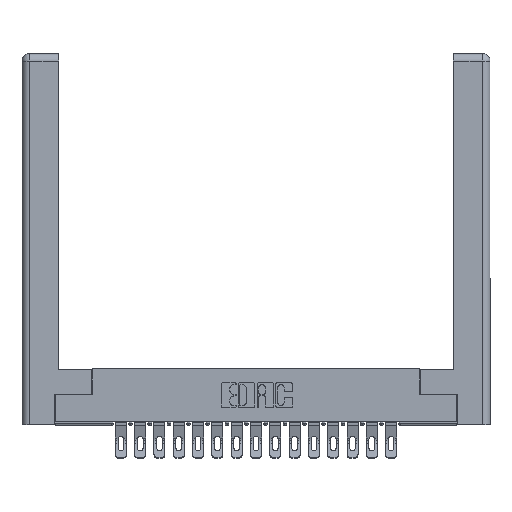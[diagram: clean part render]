
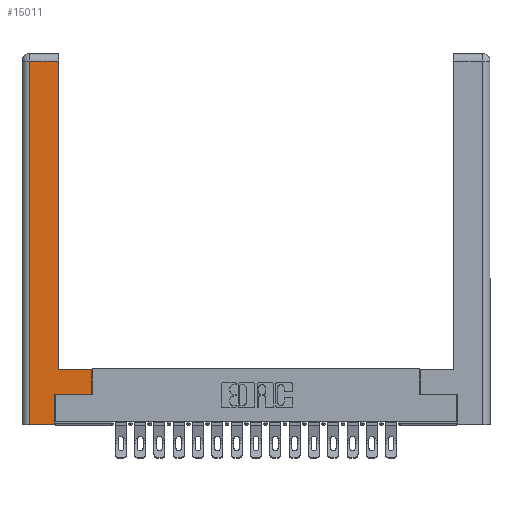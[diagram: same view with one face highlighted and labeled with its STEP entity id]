
A CAD part, top view. The second image highlights one B-rep face of the part: STEP entity #15011.
In plain terms, the highlighted planar face has unit normal (0, 0, 1).
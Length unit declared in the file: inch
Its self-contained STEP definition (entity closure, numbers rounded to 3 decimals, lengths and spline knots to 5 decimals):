
#7 = LINE ( 'NONE', #7671, #4098 ) ;
#144 = VECTOR ( 'NONE', #14500, 39.37008 ) ;
#373 = CARTESIAN_POINT ( 'NONE',  ( 0.565, 0.245, 0. ) ) ;
#655 = VERTEX_POINT ( 'NONE', #14239 ) ;
#1363 = ORIENTED_EDGE ( 'NONE', *, *, #14459, .T. ) ;
#1919 = EDGE_CURVE ( 'NONE', #4207, #3545, #17391, .T. ) ;
#2117 = ORIENTED_EDGE ( 'NONE', *, *, #2581, .T. ) ;
#2527 = DIRECTION ( 'NONE',  ( 1., 0., 0. ) ) ;
#2581 = EDGE_CURVE ( 'NONE', #3545, #7772, #22060, .T. ) ;
#2795 = VECTOR ( 'NONE', #2527, 39.37008 ) ;
#3545 = VERTEX_POINT ( 'NONE', #6510 ) ;
#3622 = VERTEX_POINT ( 'NONE', #15673 ) ;
#3811 = CARTESIAN_POINT ( 'NONE',  ( 0.0615, 0., 0. ) ) ;
#3908 = EDGE_CURVE ( 'NONE', #19692, #655, #21879, .T. ) ;
#4098 = VECTOR ( 'NONE', #12976, 39.37008 ) ;
#4207 = VERTEX_POINT ( 'NONE', #6625 ) ;
#5634 = LINE ( 'NONE', #19625, #15302 ) ;
#5689 = DIRECTION ( 'NONE',  ( -1., 0., 0. ) ) ;
#6510 = CARTESIAN_POINT ( 'NONE',  ( 0.295, 2.94, 0. ) ) ;
#6583 = DIRECTION ( 'NONE',  ( 0., 1., 0. ) ) ;
#6625 = CARTESIAN_POINT ( 'NONE',  ( 0.295, 0.45, 0. ) ) ;
#6927 = EDGE_CURVE ( 'NONE', #14269, #19692, #21484, .T. ) ;
#7187 = ORIENTED_EDGE ( 'NONE', *, *, #1919, .T. ) ;
#7305 = ORIENTED_EDGE ( 'NONE', *, *, #6927, .T. ) ;
#7671 = CARTESIAN_POINT ( 'NONE',  ( 0.265, 0.245, 0. ) ) ;
#7772 = VERTEX_POINT ( 'NONE', #12372 ) ;
#8461 = ORIENTED_EDGE ( 'NONE', *, *, #19697, .T. ) ;
#8891 = VECTOR ( 'NONE', #6583, 39.37008 ) ;
#9473 = EDGE_CURVE ( 'NONE', #20673, #14269, #7, .T. ) ;
#12002 = DIRECTION ( 'NONE',  ( 1., 0., 0. ) ) ;
#12237 = LINE ( 'NONE', #16715, #2795 ) ;
#12372 = CARTESIAN_POINT ( 'NONE',  ( 0.0615, 2.94, 0. ) ) ;
#12428 = CARTESIAN_POINT ( 'NONE',  ( 0.265, 0.245, 0. ) ) ;
#12960 = VECTOR ( 'NONE', #12002, 39.37008 ) ;
#12976 = DIRECTION ( 'NONE',  ( 0., 1., 0. ) ) ;
#13208 = EDGE_LOOP ( 'NONE', ( #7187, #2117, #1363, #18800, #18026, #7305, #19534, #8461 ) ) ;
#14239 = CARTESIAN_POINT ( 'NONE',  ( 0.565, 0.45, 0. ) ) ;
#14269 = VERTEX_POINT ( 'NONE', #12428 ) ;
#14459 = EDGE_CURVE ( 'NONE', #7772, #3622, #14745, .T. ) ;
#14472 = FACE_OUTER_BOUND ( 'NONE', #13208, .T. ) ;
#14500 = DIRECTION ( 'NONE',  ( 0., -1., 0. ) ) ;
#14745 = LINE ( 'NONE', #3811, #144 ) ;
#15011 = ADVANCED_FACE ( 'NONE', ( #14472 ), #16556, .F. ) ;
#15013 = EDGE_CURVE ( 'NONE', #3622, #20673, #12237, .T. ) ;
#15295 = CARTESIAN_POINT ( 'NONE',  ( 0.265, 0., 0. ) ) ;
#15302 = VECTOR ( 'NONE', #5689, 39.37008 ) ;
#15673 = CARTESIAN_POINT ( 'NONE',  ( 0.0615, 0., 0. ) ) ;
#15733 = VECTOR ( 'NONE', #21036, 39.37008 ) ;
#16556 = PLANE ( 'NONE',  #19281 ) ;
#16715 = CARTESIAN_POINT ( 'NONE',  ( 0.265, 0., 0. ) ) ;
#17207 = CARTESIAN_POINT ( 'NONE',  ( 0.565, 0.245, 0. ) ) ;
#17254 = CARTESIAN_POINT ( 'NONE',  ( 0.295, 3., 0. ) ) ;
#17288 = CARTESIAN_POINT ( 'NONE',  ( 0.0615, 2.94, 0. ) ) ;
#17373 = VECTOR ( 'NONE', #22593, 39.37008 ) ;
#17391 = LINE ( 'NONE', #17254, #15733 ) ;
#18026 = ORIENTED_EDGE ( 'NONE', *, *, #9473, .T. ) ;
#18264 = DIRECTION ( 'NONE',  ( 0., 0., -1. ) ) ;
#18800 = ORIENTED_EDGE ( 'NONE', *, *, #15013, .T. ) ;
#19281 = AXIS2_PLACEMENT_3D ( 'NONE', #20187, #18264, #21824 ) ;
#19534 = ORIENTED_EDGE ( 'NONE', *, *, #3908, .T. ) ;
#19625 = CARTESIAN_POINT ( 'NONE',  ( 0.295, 0.45, 0. ) ) ;
#19692 = VERTEX_POINT ( 'NONE', #373 ) ;
#19697 = EDGE_CURVE ( 'NONE', #655, #4207, #5634, .T. ) ;
#20187 = CARTESIAN_POINT ( 'NONE',  ( 0., 0., 0. ) ) ;
#20515 = CARTESIAN_POINT ( 'NONE',  ( 0.565, 0.45, 0. ) ) ;
#20673 = VERTEX_POINT ( 'NONE', #15295 ) ;
#21036 = DIRECTION ( 'NONE',  ( 0., 1., 0. ) ) ;
#21484 = LINE ( 'NONE', #17207, #12960 ) ;
#21824 = DIRECTION ( 'NONE',  ( -1., 0., 0. ) ) ;
#21879 = LINE ( 'NONE', #20515, #8891 ) ;
#22060 = LINE ( 'NONE', #17288, #17373 ) ;
#22593 = DIRECTION ( 'NONE',  ( -1., 0., 0. ) ) ;
